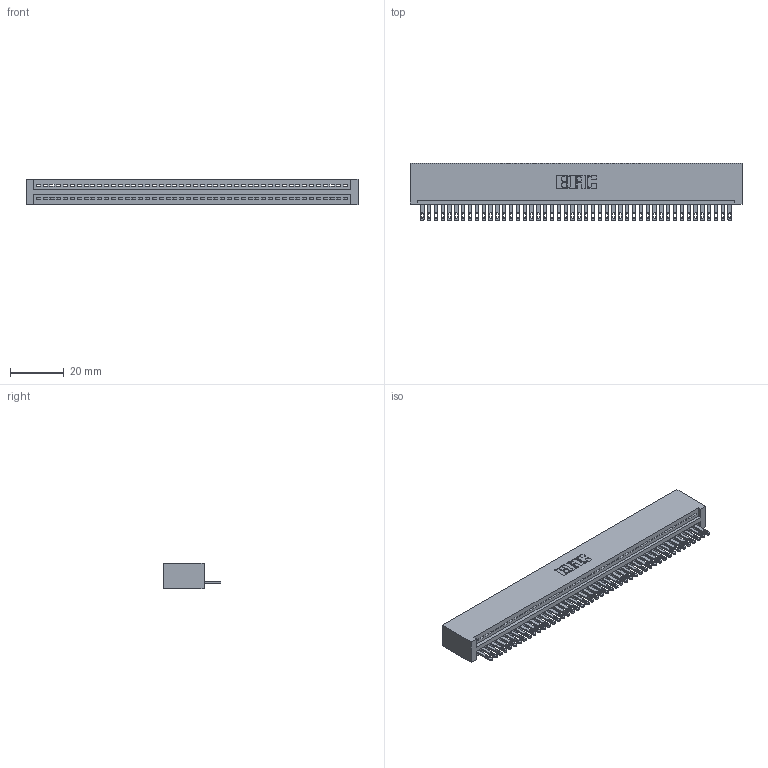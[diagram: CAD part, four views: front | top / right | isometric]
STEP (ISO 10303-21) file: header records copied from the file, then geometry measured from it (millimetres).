
FILE_DESCRIPTION (( 'STEP AP203' ), '1' );
FILE_NAME ('895-046-500-101.STEP', '2020-09-27T04:32:20', ( '' ), ( '' ), 'SwSTEP 2.0', 'SolidWorks 2020', '' );
FILE_SCHEMA (( 'CONFIG_CONTROL_DESIGN' ));
Length unit declared in the file: inch
Products named in the file (3): 895-046-500-101; 345-292-001_345-293-100; 845 Part_No Mounting Lugs
Assembly tree (47 placements, depth 2):
  895-046-500-101
    845 Part_No Mounting Lugs
    345-292-001_345-293-100  x46
Bounding box: 123.44 x 21.51 x 9.4 mm (x, y, z)
Volume: 12370.4 mm3; surface area: 16787 mm2
Topology: 47 solids, 47 shells, 2602 faces, 8045 edges, 5362 vertices
Faces by surface type: plane 1640, cylinder 962
Entity records: 33735 total; most frequent: CARTESIAN_POINT 5850, ORIENTED_EDGE 5830, DIRECTION 5099, EDGE_CURVE 2915, LINE 2603, VECTOR 2603, VERTEX_POINT 1942, AXIS2_PLACEMENT_3D 1248
